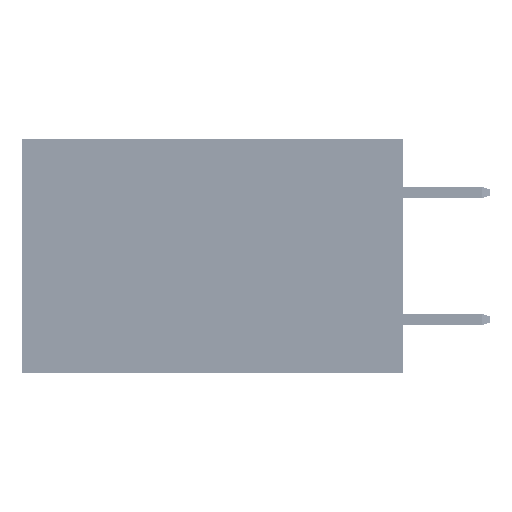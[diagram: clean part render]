
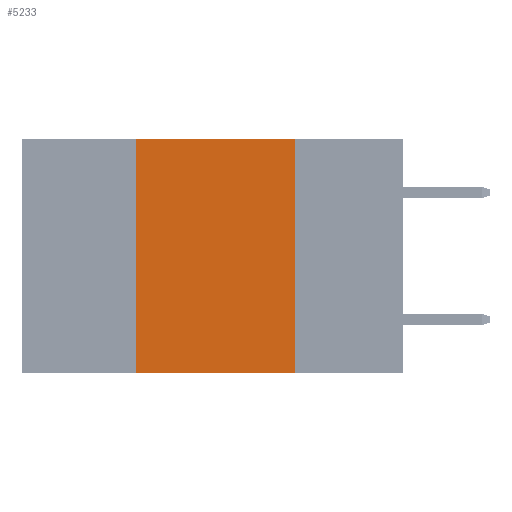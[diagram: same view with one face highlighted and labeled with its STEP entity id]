
A CAD part, left-side view. The second image highlights one B-rep face of the part: STEP entity #5233.
In plain terms, the highlighted planar face has unit normal (-1, 0, 0).
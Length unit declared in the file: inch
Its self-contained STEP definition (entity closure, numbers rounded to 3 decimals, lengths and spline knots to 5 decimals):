
#891 = PLANE ( 'NONE',  #20430 ) ;
#1572 = CARTESIAN_POINT ( 'NONE',  ( 0., 0.42, 0. ) ) ;
#1661 = VERTEX_POINT ( 'NONE', #4620 ) ;
#3331 = VECTOR ( 'NONE', #41119, 39.37008 ) ;
#4534 = VECTOR ( 'NONE', #5749, 39.37008 ) ;
#4620 = CARTESIAN_POINT ( 'NONE',  ( 0., 0.17, 0. ) ) ;
#5233 = ADVANCED_FACE ( 'NONE', ( #15752 ), #891, .F. ) ;
#5273 = LINE ( 'NONE', #12806, #4534 ) ;
#5749 = DIRECTION ( 'NONE',  ( 0., 0., -1. ) ) ;
#10229 = VECTOR ( 'NONE', #37956, 39.37008 ) ;
#10868 = LINE ( 'NONE', #25767, #3331 ) ;
#12806 = CARTESIAN_POINT ( 'NONE',  ( 0., 0.17, 0. ) ) ;
#13261 = EDGE_CURVE ( 'NONE', #1661, #30121, #5273, .T. ) ;
#14980 = ORIENTED_EDGE ( 'NONE', *, *, #30508, .F. ) ;
#15468 = VERTEX_POINT ( 'NONE', #32337 ) ;
#15752 = FACE_OUTER_BOUND ( 'NONE', #34925, .T. ) ;
#16458 = CARTESIAN_POINT ( 'NONE',  ( 0., 0.6, -0.37 ) ) ;
#16670 = LINE ( 'NONE', #1572, #38674 ) ;
#20430 = AXIS2_PLACEMENT_3D ( 'NONE', #30637, #45498, #42090 ) ;
#25767 = CARTESIAN_POINT ( 'NONE',  ( 0., 0.6, 0. ) ) ;
#27166 = DIRECTION ( 'NONE',  ( 0., 0., 1. ) ) ;
#30121 = VERTEX_POINT ( 'NONE', #40688 ) ;
#30377 = ORIENTED_EDGE ( 'NONE', *, *, #33964, .T. ) ;
#30508 = EDGE_CURVE ( 'NONE', #44943, #1661, #10868, .T. ) ;
#30637 = CARTESIAN_POINT ( 'NONE',  ( 0., 0.6, 0. ) ) ;
#31348 = LINE ( 'NONE', #16458, #10229 ) ;
#32090 = CARTESIAN_POINT ( 'NONE',  ( 0., 0.42, 0. ) ) ;
#32337 = CARTESIAN_POINT ( 'NONE',  ( 0., 0.42, -0.37 ) ) ;
#33964 = EDGE_CURVE ( 'NONE', #15468, #30121, #31348, .T. ) ;
#34925 = EDGE_LOOP ( 'NONE', ( #42967, #14980, #44430, #30377 ) ) ;
#37956 = DIRECTION ( 'NONE',  ( 0., -1., 0. ) ) ;
#38674 = VECTOR ( 'NONE', #27166, 39.37008 ) ;
#40688 = CARTESIAN_POINT ( 'NONE',  ( 0., 0.17, -0.37 ) ) ;
#41119 = DIRECTION ( 'NONE',  ( 0., -1., 0. ) ) ;
#42090 = DIRECTION ( 'NONE',  ( 0., 0., -1. ) ) ;
#42967 = ORIENTED_EDGE ( 'NONE', *, *, #13261, .F. ) ;
#43911 = EDGE_CURVE ( 'NONE', #15468, #44943, #16670, .T. ) ;
#44430 = ORIENTED_EDGE ( 'NONE', *, *, #43911, .F. ) ;
#44943 = VERTEX_POINT ( 'NONE', #32090 ) ;
#45498 = DIRECTION ( 'NONE',  ( 1., 0., 0. ) ) ;
